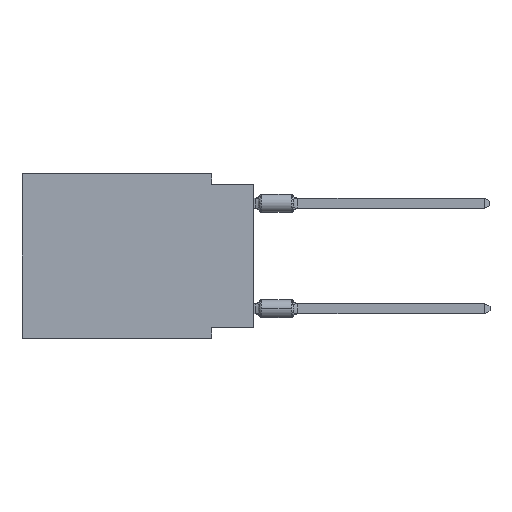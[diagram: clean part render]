
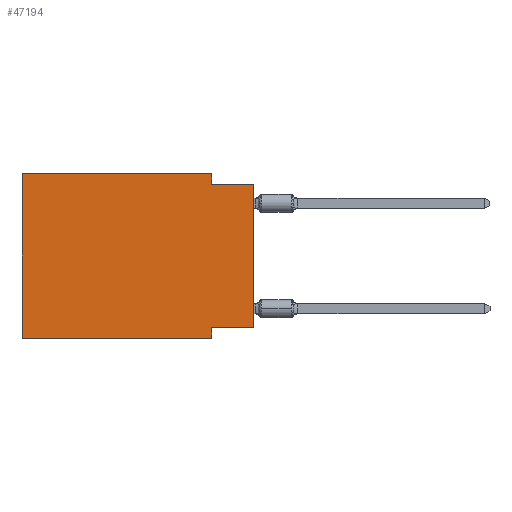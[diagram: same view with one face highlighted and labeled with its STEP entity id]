
A CAD part, left-side view. The second image highlights one B-rep face of the part: STEP entity #47194.
In plain terms, the highlighted planar face has unit normal (-1, 0, 0).
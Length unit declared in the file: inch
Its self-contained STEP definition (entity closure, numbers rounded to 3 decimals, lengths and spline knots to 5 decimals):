
#1888 = VERTEX_POINT ( 'NONE', #29081 ) ;
#2849 = VECTOR ( 'NONE', #36406, 39.37008 ) ;
#3454 = VECTOR ( 'NONE', #41470, 39.37008 ) ;
#3751 = VECTOR ( 'NONE', #34641, 39.37008 ) ;
#4830 = VECTOR ( 'NONE', #24763, 39.37008 ) ;
#5625 = ORIENTED_EDGE ( 'NONE', *, *, #30646, .T. ) ;
#6803 = CARTESIAN_POINT ( 'NONE',  ( 0., 0.1, -0.365 ) ) ;
#7747 = PLANE ( 'NONE',  #14563 ) ;
#7748 = CARTESIAN_POINT ( 'NONE',  ( 0., 0.55, 0. ) ) ;
#7895 = ORIENTED_EDGE ( 'NONE', *, *, #27239, .F. ) ;
#8065 = CARTESIAN_POINT ( 'NONE',  ( 0., 0.1, 0. ) ) ;
#8246 = DIRECTION ( 'NONE',  ( 1., 0., 0. ) ) ;
#9030 = ORIENTED_EDGE ( 'NONE', *, *, #11413, .F. ) ;
#10026 = CARTESIAN_POINT ( 'NONE',  ( 0., 0.1, -0.39 ) ) ;
#10049 = CARTESIAN_POINT ( 'NONE',  ( 0., 0.1, 0. ) ) ;
#10232 = ORIENTED_EDGE ( 'NONE', *, *, #25661, .F. ) ;
#10921 = VECTOR ( 'NONE', #29755, 39.37008 ) ;
#10931 = DIRECTION ( 'NONE',  ( 0., 0., -1. ) ) ;
#11087 = CARTESIAN_POINT ( 'NONE',  ( 0., 0.55, 0. ) ) ;
#11413 = EDGE_CURVE ( 'NONE', #12340, #42981, #30150, .T. ) ;
#12340 = VERTEX_POINT ( 'NONE', #8065 ) ;
#13040 = CARTESIAN_POINT ( 'NONE',  ( 0., 0., -0.365 ) ) ;
#13975 = EDGE_LOOP ( 'NONE', ( #5625, #47787, #9030, #7895, #22312, #20679, #47242, #10232 ) ) ;
#14299 = VERTEX_POINT ( 'NONE', #10026 ) ;
#14563 = AXIS2_PLACEMENT_3D ( 'NONE', #23708, #8246, #39902 ) ;
#17124 = VERTEX_POINT ( 'NONE', #13040 ) ;
#18502 = EDGE_CURVE ( 'NONE', #40693, #14299, #30510, .T. ) ;
#19384 = LINE ( 'NONE', #37477, #10921 ) ;
#20636 = VERTEX_POINT ( 'NONE', #38874 ) ;
#20679 = ORIENTED_EDGE ( 'NONE', *, *, #33325, .T. ) ;
#20708 = CARTESIAN_POINT ( 'NONE',  ( 0., 0.55, 0. ) ) ;
#22312 = ORIENTED_EDGE ( 'NONE', *, *, #50499, .F. ) ;
#23705 = DIRECTION ( 'NONE',  ( 0., 0., 1. ) ) ;
#23708 = CARTESIAN_POINT ( 'NONE',  ( 0., 0.55, 0. ) ) ;
#24210 = FACE_OUTER_BOUND ( 'NONE', #13975, .T. ) ;
#24763 = DIRECTION ( 'NONE',  ( 0., -1., 0. ) ) ;
#24998 = CARTESIAN_POINT ( 'NONE',  ( 0., 0.55, -0.39 ) ) ;
#25035 = LINE ( 'NONE', #44567, #4830 ) ;
#25661 = EDGE_CURVE ( 'NONE', #17124, #40693, #19384, .T. ) ;
#27057 = VECTOR ( 'NONE', #23705, 39.37008 ) ;
#27239 = EDGE_CURVE ( 'NONE', #36495, #12340, #28709, .T. ) ;
#27586 = LINE ( 'NONE', #11087, #27057 ) ;
#28709 = LINE ( 'NONE', #20708, #2849 ) ;
#29081 = CARTESIAN_POINT ( 'NONE',  ( 0., 0., -0.025 ) ) ;
#29755 = DIRECTION ( 'NONE',  ( 0., 1., 0. ) ) ;
#30150 = LINE ( 'NONE', #10049, #3454 ) ;
#30510 = LINE ( 'NONE', #46175, #38305 ) ;
#30646 = EDGE_CURVE ( 'NONE', #17124, #1888, #46720, .T. ) ;
#33325 = EDGE_CURVE ( 'NONE', #20636, #14299, #37060, .T. ) ;
#34641 = DIRECTION ( 'NONE',  ( 0., 0., 1. ) ) ;
#36406 = DIRECTION ( 'NONE',  ( 0., -1., 0. ) ) ;
#36495 = VERTEX_POINT ( 'NONE', #7748 ) ;
#36762 = CARTESIAN_POINT ( 'NONE',  ( 0., 0.1, -0.025 ) ) ;
#36821 = DIRECTION ( 'NONE',  ( 0., -1., 0. ) ) ;
#37060 = LINE ( 'NONE', #24998, #43639 ) ;
#37477 = CARTESIAN_POINT ( 'NONE',  ( 0., 0., -0.365 ) ) ;
#38305 = VECTOR ( 'NONE', #10931, 39.37008 ) ;
#38874 = CARTESIAN_POINT ( 'NONE',  ( 0., 0.55, -0.39 ) ) ;
#39902 = DIRECTION ( 'NONE',  ( 0., 0., -1. ) ) ;
#40693 = VERTEX_POINT ( 'NONE', #6803 ) ;
#41470 = DIRECTION ( 'NONE',  ( 0., 0., -1. ) ) ;
#42981 = VERTEX_POINT ( 'NONE', #36762 ) ;
#43639 = VECTOR ( 'NONE', #36821, 39.37008 ) ;
#44567 = CARTESIAN_POINT ( 'NONE',  ( 0., 0., -0.025 ) ) ;
#45956 = CARTESIAN_POINT ( 'NONE',  ( 0., 0., 0. ) ) ;
#46175 = CARTESIAN_POINT ( 'NONE',  ( 0., 0.1, -0.39 ) ) ;
#46720 = LINE ( 'NONE', #45956, #3751 ) ;
#47194 = ADVANCED_FACE ( 'NONE', ( #24210 ), #7747, .F. ) ;
#47242 = ORIENTED_EDGE ( 'NONE', *, *, #18502, .F. ) ;
#47787 = ORIENTED_EDGE ( 'NONE', *, *, #50195, .F. ) ;
#50195 = EDGE_CURVE ( 'NONE', #42981, #1888, #25035, .T. ) ;
#50499 = EDGE_CURVE ( 'NONE', #20636, #36495, #27586, .T. ) ;
